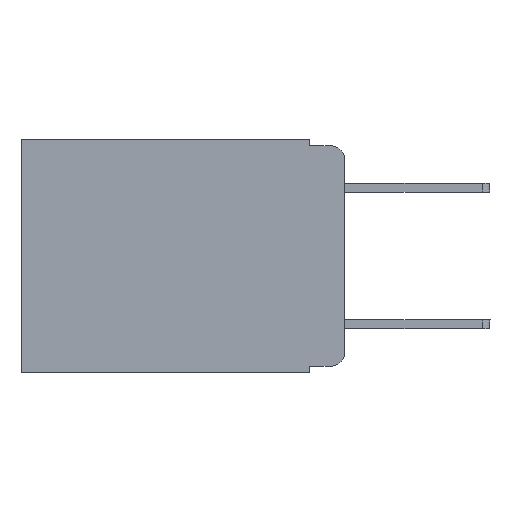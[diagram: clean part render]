
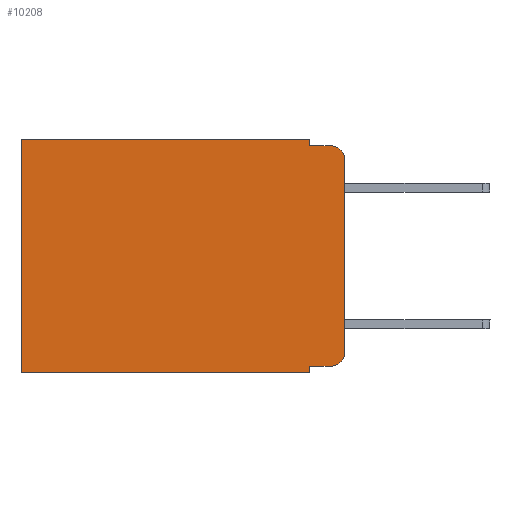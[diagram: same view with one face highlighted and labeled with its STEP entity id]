
A CAD part, left-side view. The second image highlights one B-rep face of the part: STEP entity #10208.
In plain terms, the highlighted planar face has unit normal (-1, 0, 0).
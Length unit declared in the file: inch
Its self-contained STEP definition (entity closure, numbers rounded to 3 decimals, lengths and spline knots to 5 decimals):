
#165 = ORIENTED_EDGE ( 'NONE', *, *, #3407, .T. ) ;
#359 = EDGE_CURVE ( 'NONE', #2360, #11908, #3654, .T. ) ;
#477 = DIRECTION ( 'NONE',  ( 0., 0., -1. ) ) ;
#649 = ORIENTED_EDGE ( 'NONE', *, *, #11066, .T. ) ;
#682 = AXIS2_PLACEMENT_3D ( 'NONE', #1651, #5486, #6574 ) ;
#768 = AXIS2_PLACEMENT_3D ( 'NONE', #858, #5840, #11377 ) ;
#858 = CARTESIAN_POINT ( 'NONE',  ( 0.298, 0.02, -0.03 ) ) ;
#872 = DIRECTION ( 'NONE',  ( 0., 0., -1. ) ) ;
#883 = PLANE ( 'NONE',  #5406 ) ;
#913 = CARTESIAN_POINT ( 'NONE',  ( 0.298, 0.051, -0.333 ) ) ;
#936 = CARTESIAN_POINT ( 'NONE',  ( 0.298, 0.051, 0. ) ) ;
#1030 = ORIENTED_EDGE ( 'NONE', *, *, #7123, .F. ) ;
#1120 = VERTEX_POINT ( 'NONE', #10110 ) ;
#1269 = CARTESIAN_POINT ( 'NONE',  ( 0.298, 0., 0. ) ) ;
#1575 = LINE ( 'NONE', #12220, #10832 ) ;
#1651 = CARTESIAN_POINT ( 'NONE',  ( 0.298, 0.02, -0.313 ) ) ;
#1706 = DIRECTION ( 'NONE',  ( 0., 0., -1. ) ) ;
#1829 = LINE ( 'NONE', #4830, #7413 ) ;
#1989 = VECTOR ( 'NONE', #477, 39.37008 ) ;
#2360 = VERTEX_POINT ( 'NONE', #3369 ) ;
#2370 = ORIENTED_EDGE ( 'NONE', *, *, #9993, .T. ) ;
#2399 = ORIENTED_EDGE ( 'NONE', *, *, #6738, .T. ) ;
#2593 = DIRECTION ( 'NONE',  ( 0., -1., 0. ) ) ;
#2630 = VERTEX_POINT ( 'NONE', #11712 ) ;
#2774 = VECTOR ( 'NONE', #1706, 39.37008 ) ;
#2817 = CARTESIAN_POINT ( 'NONE',  ( 0.298, 0.051, 0. ) ) ;
#3078 = EDGE_CURVE ( 'NONE', #8878, #3751, #1829, .T. ) ;
#3204 = DIRECTION ( 'NONE',  ( 0., 1., 0. ) ) ;
#3369 = CARTESIAN_POINT ( 'NONE',  ( 0.298, 0.051, -0.333 ) ) ;
#3407 = EDGE_CURVE ( 'NONE', #1120, #10782, #5600, .T. ) ;
#3654 = LINE ( 'NONE', #936, #2774 ) ;
#3751 = VERTEX_POINT ( 'NONE', #6209 ) ;
#3758 = LINE ( 'NONE', #2817, #9510 ) ;
#3847 = FACE_OUTER_BOUND ( 'NONE', #9580, .T. ) ;
#4714 = DIRECTION ( 'NONE',  ( 1., 0., 0. ) ) ;
#4718 = CARTESIAN_POINT ( 'NONE',  ( 0.298, 0.02, -0.333 ) ) ;
#4830 = CARTESIAN_POINT ( 'NONE',  ( 0.298, 0.473, 0. ) ) ;
#5406 = AXIS2_PLACEMENT_3D ( 'NONE', #8429, #4714, #11405 ) ;
#5486 = DIRECTION ( 'NONE',  ( -1., 0., 0. ) ) ;
#5600 = CIRCLE ( 'NONE', #768, 0.02 ) ;
#5705 = LINE ( 'NONE', #913, #8711 ) ;
#5840 = DIRECTION ( 'NONE',  ( -1., 0., 0. ) ) ;
#5887 = LINE ( 'NONE', #1269, #7864 ) ;
#5901 = VERTEX_POINT ( 'NONE', #5995 ) ;
#5995 = CARTESIAN_POINT ( 'NONE',  ( 0.298, 0.051, 0. ) ) ;
#6209 = CARTESIAN_POINT ( 'NONE',  ( 0.298, 0.473, -0.343 ) ) ;
#6574 = DIRECTION ( 'NONE',  ( 0., 0., -1. ) ) ;
#6738 = EDGE_CURVE ( 'NONE', #11407, #12489, #8178, .T. ) ;
#7123 = EDGE_CURVE ( 'NONE', #2630, #10782, #1575, .T. ) ;
#7142 = ORIENTED_EDGE ( 'NONE', *, *, #9051, .F. ) ;
#7413 = VECTOR ( 'NONE', #10694, 39.37008 ) ;
#7420 = EDGE_CURVE ( 'NONE', #11908, #3751, #10129, .T. ) ;
#7831 = CARTESIAN_POINT ( 'NONE',  ( 0.298, 0.473, 0. ) ) ;
#7864 = VECTOR ( 'NONE', #10907, 39.37008 ) ;
#8088 = LINE ( 'NONE', #11950, #1989 ) ;
#8166 = CARTESIAN_POINT ( 'NONE',  ( 0.298, 0., -0.343 ) ) ;
#8178 = CIRCLE ( 'NONE', #682, 0.02 ) ;
#8386 = VECTOR ( 'NONE', #3204, 39.37008 ) ;
#8429 = CARTESIAN_POINT ( 'NONE',  ( 0.298, 0., 0. ) ) ;
#8654 = DIRECTION ( 'NONE',  ( 0., -1., 0. ) ) ;
#8711 = VECTOR ( 'NONE', #8654, 39.37008 ) ;
#8878 = VERTEX_POINT ( 'NONE', #7831 ) ;
#9041 = ORIENTED_EDGE ( 'NONE', *, *, #10595, .F. ) ;
#9051 = EDGE_CURVE ( 'NONE', #1120, #12489, #8088, .T. ) ;
#9510 = VECTOR ( 'NONE', #872, 39.37008 ) ;
#9580 = EDGE_LOOP ( 'NONE', ( #7142, #165, #1030, #9041, #2370, #11162, #10214, #10758, #649, #2399 ) ) ;
#9993 = EDGE_CURVE ( 'NONE', #5901, #8878, #5887, .T. ) ;
#10110 = CARTESIAN_POINT ( 'NONE',  ( 0.298, 0., -0.03 ) ) ;
#10129 = LINE ( 'NONE', #8166, #8386 ) ;
#10208 = ADVANCED_FACE ( 'NONE', ( #3847 ), #883, .F. ) ;
#10214 = ORIENTED_EDGE ( 'NONE', *, *, #7420, .F. ) ;
#10595 = EDGE_CURVE ( 'NONE', #5901, #2630, #3758, .T. ) ;
#10694 = DIRECTION ( 'NONE',  ( 0., 0., -1. ) ) ;
#10758 = ORIENTED_EDGE ( 'NONE', *, *, #359, .F. ) ;
#10782 = VERTEX_POINT ( 'NONE', #11883 ) ;
#10832 = VECTOR ( 'NONE', #2593, 39.37008 ) ;
#10907 = DIRECTION ( 'NONE',  ( 0., 1., 0. ) ) ;
#11066 = EDGE_CURVE ( 'NONE', #2360, #11407, #5705, .T. ) ;
#11162 = ORIENTED_EDGE ( 'NONE', *, *, #3078, .T. ) ;
#11377 = DIRECTION ( 'NONE',  ( 0., 0., -1. ) ) ;
#11405 = DIRECTION ( 'NONE',  ( 0., 0., -1. ) ) ;
#11407 = VERTEX_POINT ( 'NONE', #4718 ) ;
#11635 = CARTESIAN_POINT ( 'NONE',  ( 0.298, 0.051, -0.343 ) ) ;
#11712 = CARTESIAN_POINT ( 'NONE',  ( 0.298, 0.051, -0.01 ) ) ;
#11883 = CARTESIAN_POINT ( 'NONE',  ( 0.298, 0.02, -0.01 ) ) ;
#11908 = VERTEX_POINT ( 'NONE', #11635 ) ;
#11950 = CARTESIAN_POINT ( 'NONE',  ( 0.298, 0., 0. ) ) ;
#12220 = CARTESIAN_POINT ( 'NONE',  ( 0.298, 0.051, -0.01 ) ) ;
#12381 = CARTESIAN_POINT ( 'NONE',  ( 0.298, 0., -0.313 ) ) ;
#12489 = VERTEX_POINT ( 'NONE', #12381 ) ;
